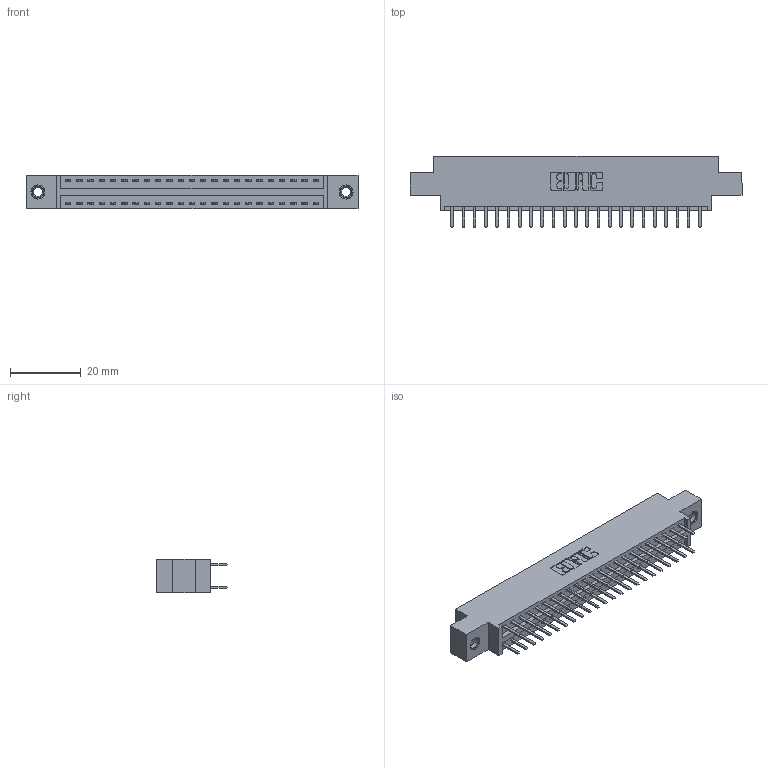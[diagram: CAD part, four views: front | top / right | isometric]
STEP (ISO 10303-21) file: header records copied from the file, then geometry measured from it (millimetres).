
FILE_DESCRIPTION (( 'STEP AP203' ), '1' );
FILE_NAME ('346-046-520-807.STEP', '2022-05-20T19:32:35', ( '' ), ( '' ), 'SwSTEP 2.0', 'SolidWorks 2020', '' );
FILE_SCHEMA (( 'CONFIG_CONTROL_DESIGN' ));
Length unit declared in the file: inch
Products named in the file (4): 346 Part_0.170 Offset - 0.156 Dia-TI; 346-046-520-807; 345-250-001_345-250-005-103; 345-292-001_345-293-120
Assembly tree (49 placements, depth 2):
  346-046-520-807
    346 Part_0.170 Offset - 0.156 Dia-TI
    345-292-001_345-293-120  x46
    345-250-001_345-250-005-103  x2
Bounding box: 93.6 x 20.02 x 9.4 mm (x, y, z)
Volume: 8791.1 mm3; surface area: 11951.4 mm2
Topology: 49 solids, 49 shells, 2762 faces, 7975 edges, 5186 vertices
Faces by surface type: plane 1814, cylinder 932, cone 12, torus 4
Entity records: 19000 total; most frequent: CARTESIAN_POINT 3155, ORIENTED_EDGE 3070, DIRECTION 2845, EDGE_CURVE 1535, LINE 1287, VECTOR 1287, VERTEX_POINT 1016, AXIS2_PLACEMENT_3D 779
